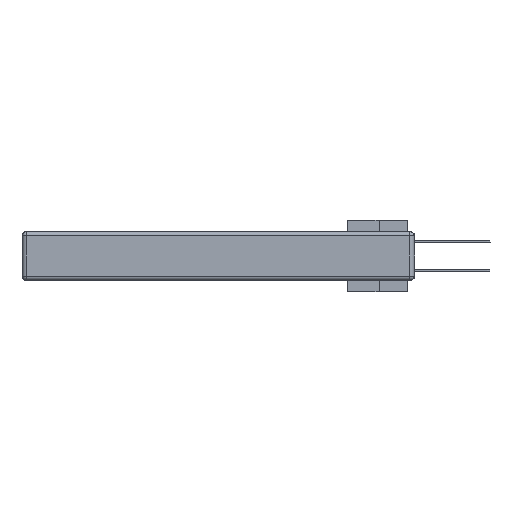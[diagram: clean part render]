
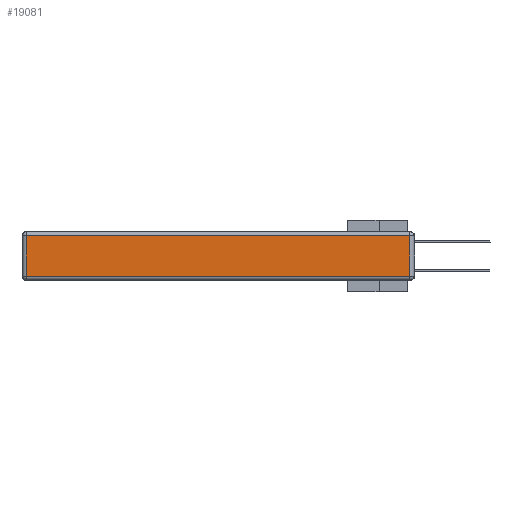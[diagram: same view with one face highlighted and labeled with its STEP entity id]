
A CAD part, left-side view. The second image highlights one B-rep face of the part: STEP entity #19081.
In plain terms, the highlighted planar face has unit normal (-1, 0, 0).
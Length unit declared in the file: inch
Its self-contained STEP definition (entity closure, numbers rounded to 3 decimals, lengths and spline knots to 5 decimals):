
#1051 = EDGE_CURVE ( 'NONE', #7245, #3997, #27679, .T. ) ;
#1464 = FACE_OUTER_BOUND ( 'NONE', #8353, .T. ) ;
#1796 = LINE ( 'NONE', #31216, #37647 ) ;
#2005 = VERTEX_POINT ( 'NONE', #9280 ) ;
#2388 = CARTESIAN_POINT ( 'NONE',  ( 0., 0., -0.343 ) ) ;
#2976 = VECTOR ( 'NONE', #24217, 39.37008 ) ;
#3182 = EDGE_CURVE ( 'NONE', #3997, #2005, #1796, .T. ) ;
#3997 = VERTEX_POINT ( 'NONE', #31975 ) ;
#6535 = CARTESIAN_POINT ( 'NONE',  ( 0., 0.03, -0.313 ) ) ;
#7033 = DIRECTION ( 'NONE',  ( 0., 0., 1. ) ) ;
#7245 = VERTEX_POINT ( 'NONE', #14621 ) ;
#8353 = EDGE_LOOP ( 'NONE', ( #39798, #38248, #35919, #20328 ) ) ;
#8756 = VERTEX_POINT ( 'NONE', #6535 ) ;
#9280 = CARTESIAN_POINT ( 'NONE',  ( 0., 2.72, -0.313 ) ) ;
#10334 = EDGE_CURVE ( 'NONE', #2005, #8756, #30501, .T. ) ;
#14621 = CARTESIAN_POINT ( 'NONE',  ( 0., 0.03, -0.03 ) ) ;
#14967 = PLANE ( 'NONE',  #26410 ) ;
#16769 = CARTESIAN_POINT ( 'NONE',  ( 0., 0., -0.313 ) ) ;
#17899 = VECTOR ( 'NONE', #35640, 39.37008 ) ;
#19081 = ADVANCED_FACE ( 'NONE', ( #1464 ), #14967, .T. ) ;
#20328 = ORIENTED_EDGE ( 'NONE', *, *, #3182, .T. ) ;
#21883 = VECTOR ( 'NONE', #7033, 39.37008 ) ;
#24217 = DIRECTION ( 'NONE',  ( 0., 1., 0. ) ) ;
#26410 = AXIS2_PLACEMENT_3D ( 'NONE', #2388, #33285, #33836 ) ;
#27679 = LINE ( 'NONE', #30820, #2976 ) ;
#28632 = CARTESIAN_POINT ( 'NONE',  ( 0., 0.03, -0.343 ) ) ;
#30501 = LINE ( 'NONE', #16769, #17899 ) ;
#30820 = CARTESIAN_POINT ( 'NONE',  ( 0., 2.75, -0.03 ) ) ;
#31216 = CARTESIAN_POINT ( 'NONE',  ( 0., 2.72, -0.343 ) ) ;
#31975 = CARTESIAN_POINT ( 'NONE',  ( 0., 2.72, -0.03 ) ) ;
#33055 = LINE ( 'NONE', #28632, #21883 ) ;
#33285 = DIRECTION ( 'NONE',  ( -1., 0., 0. ) ) ;
#33836 = DIRECTION ( 'NONE',  ( 0., 0., 1. ) ) ;
#35640 = DIRECTION ( 'NONE',  ( 0., -1., 0. ) ) ;
#35919 = ORIENTED_EDGE ( 'NONE', *, *, #1051, .T. ) ;
#36339 = EDGE_CURVE ( 'NONE', #8756, #7245, #33055, .T. ) ;
#36821 = DIRECTION ( 'NONE',  ( 0., 0., -1. ) ) ;
#37647 = VECTOR ( 'NONE', #36821, 39.37008 ) ;
#38248 = ORIENTED_EDGE ( 'NONE', *, *, #36339, .T. ) ;
#39798 = ORIENTED_EDGE ( 'NONE', *, *, #10334, .T. ) ;
